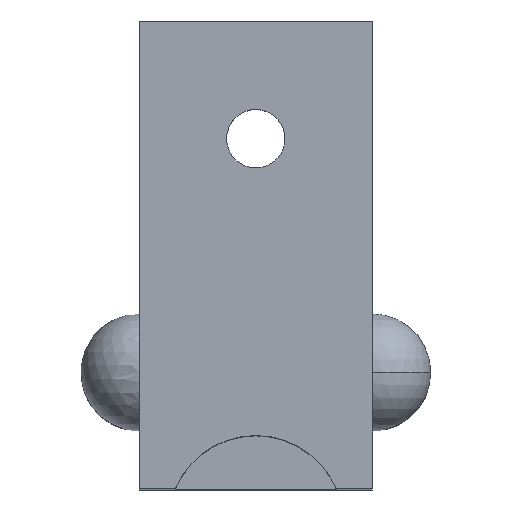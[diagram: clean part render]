
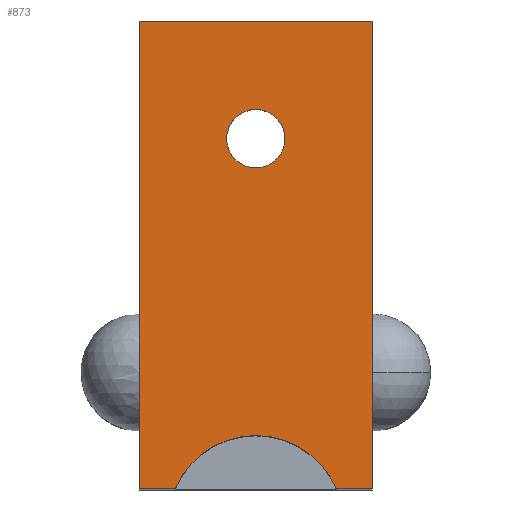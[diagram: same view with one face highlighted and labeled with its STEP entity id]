
A CAD part, top view. The second image highlights one B-rep face of the part: STEP entity #873.
In plain terms, the highlighted planar face has unit normal (0, 0, 1).
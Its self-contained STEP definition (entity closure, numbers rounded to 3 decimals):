
#5 = CARTESIAN_POINT ( 'NONE',  ( 0., 15., 15. ) ) ;
#11 = CARTESIAN_POINT ( 'NONE',  ( 0., -5., 15. ) ) ;
#19 = CARTESIAN_POINT ( 'NONE',  ( 5., 10., 15. ) ) ;
#54 = DIRECTION ( 'NONE',  ( -1., 0., 0. ) ) ;
#55 = CARTESIAN_POINT ( 'NONE',  ( 5., -6.466, 15. ) ) ;
#94 = DIRECTION ( 'NONE',  ( 1., 0., 0. ) ) ;
#96 = CARTESIAN_POINT ( 'NONE',  ( 0., -5., 15. ) ) ;
#108 = FACE_BOUND ( 'NONE', #604, .T. ) ;
#119 = FACE_OUTER_BOUND ( 'NONE', #488, .T. ) ;
#126 = CARTESIAN_POINT ( 'NONE',  ( 5., 10., 15. ) ) ;
#128 = CARTESIAN_POINT ( 'NONE',  ( 3.75, 10., 15. ) ) ;
#159 = CARTESIAN_POINT ( 'NONE',  ( 10., -5., 15. ) ) ;
#175 = VECTOR ( 'NONE', #958, 1000. ) ;
#177 = VECTOR ( 'NONE', #238, 1000. ) ;
#178 = LINE ( 'NONE', #899, #175 ) ;
#179 = VECTOR ( 'NONE', #478, 1000. ) ;
#180 = CIRCLE ( 'NONE', #443, 3.75 ) ;
#186 = LINE ( 'NONE', #159, #177 ) ;
#187 = DIRECTION ( 'NONE',  ( -1., 0., 0. ) ) ;
#188 = VECTOR ( 'NONE', #232, 1000. ) ;
#190 = LINE ( 'NONE', #805, #188 ) ;
#195 = LINE ( 'NONE', #382, #179 ) ;
#196 = CIRCLE ( 'NONE', #448, 1.25 ) ;
#202 = DIRECTION ( 'NONE',  ( -1., 0., 0. ) ) ;
#220 = VECTOR ( 'NONE', #900, 1000. ) ;
#223 = LINE ( 'NONE', #96, #220 ) ;
#232 = DIRECTION ( 'NONE',  ( -1., 0., 0. ) ) ;
#238 = DIRECTION ( 'NONE',  ( 0., -1., 0. ) ) ;
#291 = CIRCLE ( 'NONE', #503, 1.25 ) ;
#331 = PLANE ( 'NONE',  #401 ) ;
#335 = CARTESIAN_POINT ( 'NONE',  ( 10., 15., 15. ) ) ;
#347 = CARTESIAN_POINT ( 'NONE',  ( 10., -5., 15. ) ) ;
#382 = CARTESIAN_POINT ( 'NONE',  ( 10., -5., 15. ) ) ;
#401 = AXIS2_PLACEMENT_3D ( 'NONE', #412, #738, #187 ) ;
#412 = CARTESIAN_POINT ( 'NONE',  ( 10., -5., 15. ) ) ;
#427 = CARTESIAN_POINT ( 'NONE',  ( 6.25, 10., 15. ) ) ;
#429 = CARTESIAN_POINT ( 'NONE',  ( 1.549, -5., 15. ) ) ;
#443 = AXIS2_PLACEMENT_3D ( 'NONE', #55, #597, #94 ) ;
#448 = AXIS2_PLACEMENT_3D ( 'NONE', #19, #469, #54 ) ;
#468 = ORIENTED_EDGE ( 'NONE', *, *, #778, .F. ) ;
#469 = DIRECTION ( 'NONE',  ( 0., 0., 1. ) ) ;
#478 = DIRECTION ( 'NONE',  ( -1., 0., 0. ) ) ;
#479 = VERTEX_POINT ( 'NONE', #429 ) ;
#485 = VERTEX_POINT ( 'NONE', #652 ) ;
#488 = EDGE_LOOP ( 'NONE', ( #656, #468, #693, #499, #887, #751 ) ) ;
#499 = ORIENTED_EDGE ( 'NONE', *, *, #784, .F. ) ;
#503 = AXIS2_PLACEMENT_3D ( 'NONE', #126, #763, #202 ) ;
#516 = VERTEX_POINT ( 'NONE', #427 ) ;
#581 = VERTEX_POINT ( 'NONE', #347 ) ;
#588 = VERTEX_POINT ( 'NONE', #11 ) ;
#597 = DIRECTION ( 'NONE',  ( 0., 0., 1. ) ) ;
#604 = EDGE_LOOP ( 'NONE', ( #922, #828 ) ) ;
#652 = CARTESIAN_POINT ( 'NONE',  ( 8.451, -5., 15. ) ) ;
#656 = ORIENTED_EDGE ( 'NONE', *, *, #776, .F. ) ;
#671 = EDGE_CURVE ( 'NONE', #674, #516, #291, .T. ) ;
#674 = VERTEX_POINT ( 'NONE', #128 ) ;
#693 = ORIENTED_EDGE ( 'NONE', *, *, #782, .F. ) ;
#738 = DIRECTION ( 'NONE',  ( 0., 0., -1. ) ) ;
#741 = EDGE_CURVE ( 'NONE', #881, #588, #223, .T. ) ;
#751 = ORIENTED_EDGE ( 'NONE', *, *, #741, .T. ) ;
#763 = DIRECTION ( 'NONE',  ( 0., 0., 1. ) ) ;
#774 = EDGE_CURVE ( 'NONE', #516, #674, #196, .T. ) ;
#776 = EDGE_CURVE ( 'NONE', #479, #588, #190, .T. ) ;
#778 = EDGE_CURVE ( 'NONE', #485, #479, #180, .T. ) ;
#782 = EDGE_CURVE ( 'NONE', #581, #485, #195, .T. ) ;
#784 = EDGE_CURVE ( 'NONE', #877, #581, #186, .T. ) ;
#787 = EDGE_CURVE ( 'NONE', #881, #877, #178, .T. ) ;
#805 = CARTESIAN_POINT ( 'NONE',  ( 10., -5., 15. ) ) ;
#828 = ORIENTED_EDGE ( 'NONE', *, *, #774, .F. ) ;
#873 = ADVANCED_FACE ( 'NONE', ( #108, #119 ), #331, .F. ) ;
#877 = VERTEX_POINT ( 'NONE', #335 ) ;
#881 = VERTEX_POINT ( 'NONE', #5 ) ;
#887 = ORIENTED_EDGE ( 'NONE', *, *, #787, .F. ) ;
#899 = CARTESIAN_POINT ( 'NONE',  ( 10., 15., 15. ) ) ;
#900 = DIRECTION ( 'NONE',  ( 0., -1., 0. ) ) ;
#922 = ORIENTED_EDGE ( 'NONE', *, *, #671, .F. ) ;
#958 = DIRECTION ( 'NONE',  ( 1., 0., 0. ) ) ;
